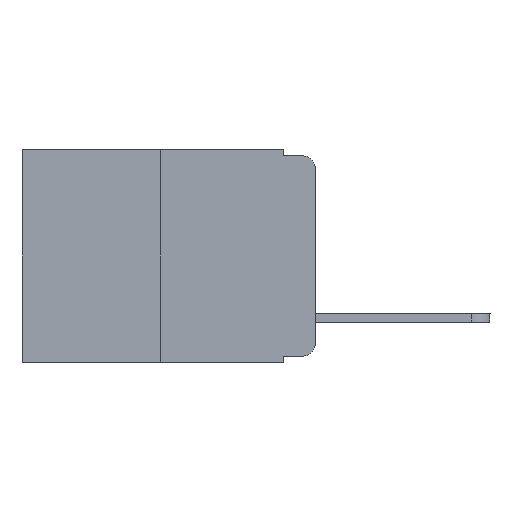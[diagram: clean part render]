
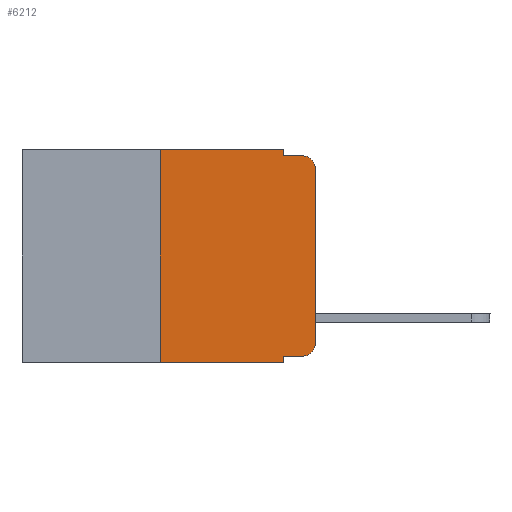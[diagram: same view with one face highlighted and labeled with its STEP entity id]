
A CAD part, left-side view. The second image highlights one B-rep face of the part: STEP entity #6212.
In plain terms, the highlighted planar face has unit normal (-1, 0, 0).
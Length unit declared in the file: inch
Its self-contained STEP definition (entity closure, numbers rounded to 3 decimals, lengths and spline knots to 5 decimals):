
#115 = EDGE_CURVE ( 'NONE', #9324, #8334, #7841, .T. ) ;
#182 = VECTOR ( 'NONE', #9054, 39.37008 ) ;
#217 = VERTEX_POINT ( 'NONE', #9367 ) ;
#524 = ORIENTED_EDGE ( 'NONE', *, *, #2996, .T. ) ;
#635 = ORIENTED_EDGE ( 'NONE', *, *, #115, .T. ) ;
#802 = LINE ( 'NONE', #3156, #1105 ) ;
#838 = VERTEX_POINT ( 'NONE', #8329 ) ;
#925 = CARTESIAN_POINT ( 'NONE',  ( 0., 0.051, -0.333 ) ) ;
#1040 = CIRCLE ( 'NONE', #6680, 0.02 ) ;
#1101 = EDGE_CURVE ( 'NONE', #217, #9739, #802, .T. ) ;
#1105 = VECTOR ( 'NONE', #2419, 39.37008 ) ;
#1183 = DIRECTION ( 'NONE',  ( 0., -1., 0. ) ) ;
#1476 = ORIENTED_EDGE ( 'NONE', *, *, #8816, .F. ) ;
#1701 = CARTESIAN_POINT ( 'NONE',  ( 0., 0.02, -0.333 ) ) ;
#1821 = CARTESIAN_POINT ( 'NONE',  ( 0., 0.051, -0.333 ) ) ;
#1837 = CARTESIAN_POINT ( 'NONE',  ( 0., 0.473, 0. ) ) ;
#1990 = DIRECTION ( 'NONE',  ( 0., 0., -1. ) ) ;
#2107 = CARTESIAN_POINT ( 'NONE',  ( 0., 0.25, 0. ) ) ;
#2161 = CARTESIAN_POINT ( 'NONE',  ( 0., 0.051, 0. ) ) ;
#2210 = CARTESIAN_POINT ( 'NONE',  ( 0., 0.02, -0.313 ) ) ;
#2419 = DIRECTION ( 'NONE',  ( 0., 0., -1. ) ) ;
#2536 = EDGE_CURVE ( 'NONE', #9324, #3649, #6600, .T. ) ;
#2593 = CARTESIAN_POINT ( 'NONE',  ( 0., 0.473, 0. ) ) ;
#2635 = LINE ( 'NONE', #2593, #8620 ) ;
#2745 = VECTOR ( 'NONE', #9616, 39.37008 ) ;
#2849 = DIRECTION ( 'NONE',  ( 0., 0., -1. ) ) ;
#2996 = EDGE_CURVE ( 'NONE', #9053, #3649, #7488, .T. ) ;
#3156 = CARTESIAN_POINT ( 'NONE',  ( 0., 0.051, 0. ) ) ;
#3231 = ORIENTED_EDGE ( 'NONE', *, *, #2536, .F. ) ;
#3338 = FACE_OUTER_BOUND ( 'NONE', #3767, .T. ) ;
#3431 = CARTESIAN_POINT ( 'NONE',  ( 0., 0.051, -0.01 ) ) ;
#3647 = ORIENTED_EDGE ( 'NONE', *, *, #1101, .F. ) ;
#3649 = VERTEX_POINT ( 'NONE', #7789 ) ;
#3767 = EDGE_LOOP ( 'NONE', ( #8409, #7600, #1476, #3647, #7530, #4125, #524, #3231, #635, #5516 ) ) ;
#3899 = DIRECTION ( 'NONE',  ( 0., -1., 0. ) ) ;
#4125 = ORIENTED_EDGE ( 'NONE', *, *, #5928, .F. ) ;
#4239 = CARTESIAN_POINT ( 'NONE',  ( 0., 0., -0.03 ) ) ;
#4252 = CARTESIAN_POINT ( 'NONE',  ( 0., 0.473, -0.343 ) ) ;
#4518 = DIRECTION ( 'NONE',  ( -1., 0., 0. ) ) ;
#4960 = LINE ( 'NONE', #2107, #8400 ) ;
#5064 = DIRECTION ( 'NONE',  ( 0., 0., 1. ) ) ;
#5095 = CARTESIAN_POINT ( 'NONE',  ( 0., 0.25, -0.343 ) ) ;
#5223 = CARTESIAN_POINT ( 'NONE',  ( 0., 0.25, 0. ) ) ;
#5482 = CIRCLE ( 'NONE', #9208, 0.02 ) ;
#5516 = ORIENTED_EDGE ( 'NONE', *, *, #8160, .T. ) ;
#5928 = EDGE_CURVE ( 'NONE', #9053, #6106, #4960, .T. ) ;
#6106 = VERTEX_POINT ( 'NONE', #5223 ) ;
#6212 = ADVANCED_FACE ( 'NONE', ( #3338 ), #9433, .F. ) ;
#6480 = AXIS2_PLACEMENT_3D ( 'NONE', #1837, #7804, #7854 ) ;
#6600 = LINE ( 'NONE', #2161, #8139 ) ;
#6680 = AXIS2_PLACEMENT_3D ( 'NONE', #2210, #4518, #9737 ) ;
#6715 = VECTOR ( 'NONE', #1183, 39.37008 ) ;
#6739 = EDGE_CURVE ( 'NONE', #6106, #217, #2635, .T. ) ;
#6775 = VERTEX_POINT ( 'NONE', #4239 ) ;
#7093 = LINE ( 'NONE', #3431, #2745 ) ;
#7397 = EDGE_CURVE ( 'NONE', #6775, #838, #5482, .T. ) ;
#7482 = CARTESIAN_POINT ( 'NONE',  ( 0., 0., 0. ) ) ;
#7488 = LINE ( 'NONE', #4252, #6715 ) ;
#7530 = ORIENTED_EDGE ( 'NONE', *, *, #6739, .F. ) ;
#7600 = ORIENTED_EDGE ( 'NONE', *, *, #7397, .T. ) ;
#7789 = CARTESIAN_POINT ( 'NONE',  ( 0., 0.051, -0.343 ) ) ;
#7804 = DIRECTION ( 'NONE',  ( 1., 0., 0. ) ) ;
#7841 = LINE ( 'NONE', #925, #9456 ) ;
#7854 = DIRECTION ( 'NONE',  ( 0., 0., -1. ) ) ;
#7922 = CARTESIAN_POINT ( 'NONE',  ( 0., 0.051, -0.01 ) ) ;
#8027 = VERTEX_POINT ( 'NONE', #8171 ) ;
#8139 = VECTOR ( 'NONE', #2849, 39.37008 ) ;
#8144 = LINE ( 'NONE', #7482, #182 ) ;
#8160 = EDGE_CURVE ( 'NONE', #8334, #8027, #1040, .T. ) ;
#8171 = CARTESIAN_POINT ( 'NONE',  ( 0., 0., -0.313 ) ) ;
#8329 = CARTESIAN_POINT ( 'NONE',  ( 0., 0.02, -0.01 ) ) ;
#8334 = VERTEX_POINT ( 'NONE', #1701 ) ;
#8400 = VECTOR ( 'NONE', #5064, 39.37008 ) ;
#8409 = ORIENTED_EDGE ( 'NONE', *, *, #9025, .T. ) ;
#8620 = VECTOR ( 'NONE', #8946, 39.37008 ) ;
#8816 = EDGE_CURVE ( 'NONE', #9739, #838, #7093, .T. ) ;
#8946 = DIRECTION ( 'NONE',  ( 0., -1., 0. ) ) ;
#8952 = DIRECTION ( 'NONE',  ( -1., 0., 0. ) ) ;
#9004 = CARTESIAN_POINT ( 'NONE',  ( 0., 0.02, -0.03 ) ) ;
#9025 = EDGE_CURVE ( 'NONE', #8027, #6775, #8144, .T. ) ;
#9053 = VERTEX_POINT ( 'NONE', #5095 ) ;
#9054 = DIRECTION ( 'NONE',  ( 0., 0., 1. ) ) ;
#9208 = AXIS2_PLACEMENT_3D ( 'NONE', #9004, #8952, #1990 ) ;
#9324 = VERTEX_POINT ( 'NONE', #1821 ) ;
#9367 = CARTESIAN_POINT ( 'NONE',  ( 0., 0.051, 0. ) ) ;
#9433 = PLANE ( 'NONE',  #6480 ) ;
#9456 = VECTOR ( 'NONE', #3899, 39.37008 ) ;
#9616 = DIRECTION ( 'NONE',  ( 0., -1., 0. ) ) ;
#9737 = DIRECTION ( 'NONE',  ( 0., 0., -1. ) ) ;
#9739 = VERTEX_POINT ( 'NONE', #7922 ) ;
